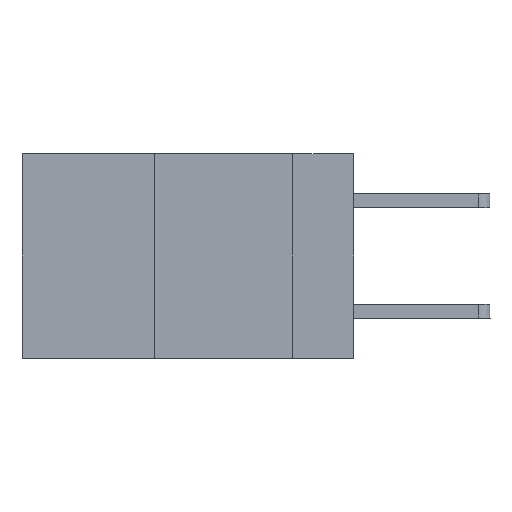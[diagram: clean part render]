
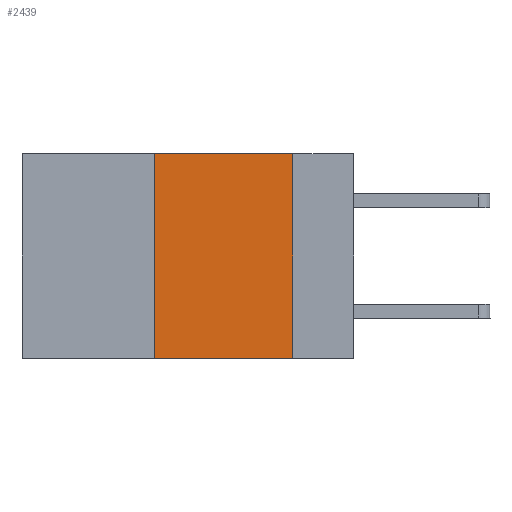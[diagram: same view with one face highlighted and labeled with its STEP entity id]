
A CAD part, left-side view. The second image highlights one B-rep face of the part: STEP entity #2439.
In plain terms, the highlighted planar face has unit normal (-1, 0, 0).
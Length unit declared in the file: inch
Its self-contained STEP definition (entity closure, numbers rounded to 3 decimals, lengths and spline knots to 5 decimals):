
#22 = DIRECTION ( 'NONE',  ( 0., -1., 0. ) ) ;
#69 = CARTESIAN_POINT ( 'NONE',  ( 0., 0.11, -0.37 ) ) ;
#481 = CARTESIAN_POINT ( 'NONE',  ( 0., 0.36, 0. ) ) ;
#561 = AXIS2_PLACEMENT_3D ( 'NONE', #4730, #1732, #6160 ) ;
#642 = ORIENTED_EDGE ( 'NONE', *, *, #670, .F. ) ;
#670 = EDGE_CURVE ( 'NONE', #2587, #6254, #2216, .T. ) ;
#1554 = DIRECTION ( 'NONE',  ( 0., 0., 1. ) ) ;
#1673 = CARTESIAN_POINT ( 'NONE',  ( 0., 0.36, -0.37 ) ) ;
#1732 = DIRECTION ( 'NONE',  ( 1., 0., 0. ) ) ;
#1817 = FACE_OUTER_BOUND ( 'NONE', #5370, .T. ) ;
#2216 = LINE ( 'NONE', #4465, #7370 ) ;
#2439 = ADVANCED_FACE ( 'NONE', ( #1817 ), #2537, .F. ) ;
#2537 = PLANE ( 'NONE',  #561 ) ;
#2587 = VERTEX_POINT ( 'NONE', #1673 ) ;
#2973 = VERTEX_POINT ( 'NONE', #69 ) ;
#3361 = CARTESIAN_POINT ( 'NONE',  ( 0., 0.6, -0.37 ) ) ;
#3645 = VERTEX_POINT ( 'NONE', #3771 ) ;
#3771 = CARTESIAN_POINT ( 'NONE',  ( 0., 0.11, 0. ) ) ;
#3812 = VECTOR ( 'NONE', #22, 39.37008 ) ;
#3955 = LINE ( 'NONE', #8091, #3812 ) ;
#3983 = ORIENTED_EDGE ( 'NONE', *, *, #7913, .T. ) ;
#4465 = CARTESIAN_POINT ( 'NONE',  ( 0., 0.36, 0. ) ) ;
#4730 = CARTESIAN_POINT ( 'NONE',  ( 0., 0.6, 0. ) ) ;
#4791 = LINE ( 'NONE', #3361, #5197 ) ;
#5173 = LINE ( 'NONE', #8774, #7606 ) ;
#5197 = VECTOR ( 'NONE', #9245, 39.37008 ) ;
#5370 = EDGE_LOOP ( 'NONE', ( #7732, #8287, #642, #3983 ) ) ;
#5737 = EDGE_CURVE ( 'NONE', #3645, #2973, #5173, .T. ) ;
#6160 = DIRECTION ( 'NONE',  ( 0., 0., -1. ) ) ;
#6197 = EDGE_CURVE ( 'NONE', #6254, #3645, #3955, .T. ) ;
#6254 = VERTEX_POINT ( 'NONE', #481 ) ;
#7370 = VECTOR ( 'NONE', #1554, 39.37008 ) ;
#7404 = DIRECTION ( 'NONE',  ( 0., 0., -1. ) ) ;
#7606 = VECTOR ( 'NONE', #7404, 39.37008 ) ;
#7732 = ORIENTED_EDGE ( 'NONE', *, *, #5737, .F. ) ;
#7913 = EDGE_CURVE ( 'NONE', #2587, #2973, #4791, .T. ) ;
#8091 = CARTESIAN_POINT ( 'NONE',  ( 0., 0.6, 0. ) ) ;
#8287 = ORIENTED_EDGE ( 'NONE', *, *, #6197, .F. ) ;
#8774 = CARTESIAN_POINT ( 'NONE',  ( 0., 0.11, 0. ) ) ;
#9245 = DIRECTION ( 'NONE',  ( 0., -1., 0. ) ) ;
